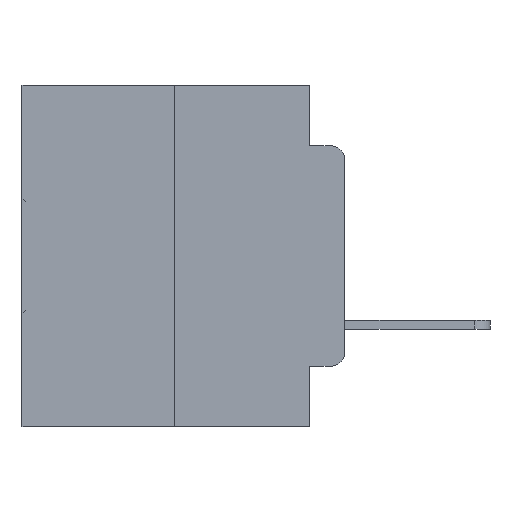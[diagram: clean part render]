
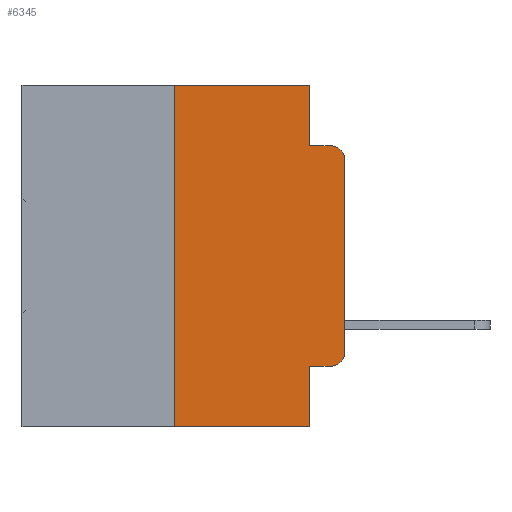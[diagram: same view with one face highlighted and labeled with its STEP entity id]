
A CAD part, left-side view. The second image highlights one B-rep face of the part: STEP entity #6345.
In plain terms, the highlighted planar face has unit normal (-1, 0, 0).
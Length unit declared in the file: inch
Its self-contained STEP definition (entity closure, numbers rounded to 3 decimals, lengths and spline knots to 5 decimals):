
#619 = VECTOR ( 'NONE', #29872, 39.37008 ) ;
#1497 = LINE ( 'NONE', #9899, #13523 ) ;
#1854 = CARTESIAN_POINT ( 'NONE',  ( 0., 0.051, 0. ) ) ;
#1888 = LINE ( 'NONE', #17918, #14671 ) ;
#1907 = LINE ( 'NONE', #19699, #21038 ) ;
#2262 = AXIS2_PLACEMENT_3D ( 'NONE', #8874, #25663, #11394 ) ;
#2297 = VERTEX_POINT ( 'NONE', #15296 ) ;
#3124 = CIRCLE ( 'NONE', #2262, 0.02 ) ;
#3326 = DIRECTION ( 'NONE',  ( 0., 0., -1. ) ) ;
#3469 = ORIENTED_EDGE ( 'NONE', *, *, #19049, .F. ) ;
#3562 = CARTESIAN_POINT ( 'NONE',  ( 0., 0.02, -0.0885 ) ) ;
#5231 = CARTESIAN_POINT ( 'NONE',  ( 0., 0., -0.3915 ) ) ;
#5654 = CARTESIAN_POINT ( 'NONE',  ( 0., 0.051, -0.0885 ) ) ;
#5661 = DIRECTION ( 'NONE',  ( 1., 0., 0. ) ) ;
#6345 = ADVANCED_FACE ( 'NONE', ( #7592 ), #18008, .F. ) ;
#6910 = CARTESIAN_POINT ( 'NONE',  ( 0., 0.25, -0.5 ) ) ;
#7188 = VERTEX_POINT ( 'NONE', #1854 ) ;
#7385 = DIRECTION ( 'NONE',  ( 0., 0., 1. ) ) ;
#7592 = FACE_OUTER_BOUND ( 'NONE', #28493, .T. ) ;
#7648 = LINE ( 'NONE', #8805, #619 ) ;
#7826 = CARTESIAN_POINT ( 'NONE',  ( 0., 0.051, -0.5 ) ) ;
#7956 = LINE ( 'NONE', #9304, #26306 ) ;
#8029 = ORIENTED_EDGE ( 'NONE', *, *, #19196, .F. ) ;
#8427 = ORIENTED_EDGE ( 'NONE', *, *, #16736, .T. ) ;
#8770 = DIRECTION ( 'NONE',  ( 0., -1., 0. ) ) ;
#8805 = CARTESIAN_POINT ( 'NONE',  ( 0., 0.051, -0.0885 ) ) ;
#8874 = CARTESIAN_POINT ( 'NONE',  ( 0., 0.02, -0.3915 ) ) ;
#9270 = DIRECTION ( 'NONE',  ( -1., 0., 0. ) ) ;
#9304 = CARTESIAN_POINT ( 'NONE',  ( 0., 0.473, 0. ) ) ;
#9899 = CARTESIAN_POINT ( 'NONE',  ( 0., 0.051, 0. ) ) ;
#10017 = ORIENTED_EDGE ( 'NONE', *, *, #19286, .F. ) ;
#10334 = VERTEX_POINT ( 'NONE', #21685 ) ;
#11394 = DIRECTION ( 'NONE',  ( 0., 0., -1. ) ) ;
#11712 = VECTOR ( 'NONE', #8770, 39.37008 ) ;
#13026 = DIRECTION ( 'NONE',  ( 0., 0., 1. ) ) ;
#13461 = DIRECTION ( 'NONE',  ( 0., -1., 0. ) ) ;
#13523 = VECTOR ( 'NONE', #24412, 39.37008 ) ;
#13687 = CARTESIAN_POINT ( 'NONE',  ( 0., 0.473, -0.5 ) ) ;
#13739 = VERTEX_POINT ( 'NONE', #20071 ) ;
#14671 = VECTOR ( 'NONE', #13026, 39.37008 ) ;
#14996 = EDGE_CURVE ( 'NONE', #10334, #7188, #7956, .T. ) ;
#15296 = CARTESIAN_POINT ( 'NONE',  ( 0., 0., -0.1085 ) ) ;
#16200 = ORIENTED_EDGE ( 'NONE', *, *, #19373, .T. ) ;
#16364 = ORIENTED_EDGE ( 'NONE', *, *, #18334, .T. ) ;
#16550 = VECTOR ( 'NONE', #13461, 39.37008 ) ;
#16667 = AXIS2_PLACEMENT_3D ( 'NONE', #23773, #9270, #26000 ) ;
#16736 = EDGE_CURVE ( 'NONE', #29200, #27399, #30792, .T. ) ;
#17242 = ORIENTED_EDGE ( 'NONE', *, *, #14996, .F. ) ;
#17918 = CARTESIAN_POINT ( 'NONE',  ( 0., 0.25, 0. ) ) ;
#18008 = PLANE ( 'NONE',  #28939 ) ;
#18196 = EDGE_CURVE ( 'NONE', #27383, #2297, #1907, .T. ) ;
#18315 = CARTESIAN_POINT ( 'NONE',  ( 0., 0.051, 0. ) ) ;
#18334 = EDGE_CURVE ( 'NONE', #2297, #19359, #23637, .T. ) ;
#18565 = ORIENTED_EDGE ( 'NONE', *, *, #18196, .T. ) ;
#18783 = EDGE_CURVE ( 'NONE', #28816, #19359, #7648, .T. ) ;
#19049 = EDGE_CURVE ( 'NONE', #7188, #28816, #1497, .T. ) ;
#19196 = EDGE_CURVE ( 'NONE', #29200, #10334, #1888, .T. ) ;
#19286 = EDGE_CURVE ( 'NONE', #20617, #27399, #30022, .T. ) ;
#19330 = EDGE_CURVE ( 'NONE', #20617, #13739, #28707, .T. ) ;
#19359 = VERTEX_POINT ( 'NONE', #3562 ) ;
#19373 = EDGE_CURVE ( 'NONE', #13739, #27383, #3124, .T. ) ;
#19699 = CARTESIAN_POINT ( 'NONE',  ( 0., 0., 0. ) ) ;
#20071 = CARTESIAN_POINT ( 'NONE',  ( 0., 0.02, -0.4115 ) ) ;
#20258 = CARTESIAN_POINT ( 'NONE',  ( 0., 0.051, -0.4115 ) ) ;
#20617 = VERTEX_POINT ( 'NONE', #20258 ) ;
#21038 = VECTOR ( 'NONE', #7385, 39.37008 ) ;
#21562 = ORIENTED_EDGE ( 'NONE', *, *, #18783, .F. ) ;
#21685 = CARTESIAN_POINT ( 'NONE',  ( 0., 0.25, 0. ) ) ;
#22782 = DIRECTION ( 'NONE',  ( 0., 0., -1. ) ) ;
#23637 = CIRCLE ( 'NONE', #16667, 0.02 ) ;
#23773 = CARTESIAN_POINT ( 'NONE',  ( 0., 0.02, -0.1085 ) ) ;
#24321 = VECTOR ( 'NONE', #3326, 39.37008 ) ;
#24412 = DIRECTION ( 'NONE',  ( 0., 0., -1. ) ) ;
#25663 = DIRECTION ( 'NONE',  ( -1., 0., 0. ) ) ;
#26000 = DIRECTION ( 'NONE',  ( 0., 0., -1. ) ) ;
#26306 = VECTOR ( 'NONE', #30276, 39.37008 ) ;
#27068 = ORIENTED_EDGE ( 'NONE', *, *, #19330, .T. ) ;
#27383 = VERTEX_POINT ( 'NONE', #5231 ) ;
#27399 = VERTEX_POINT ( 'NONE', #7826 ) ;
#28493 = EDGE_LOOP ( 'NONE', ( #18565, #16364, #21562, #3469, #17242, #8029, #8427, #10017, #27068, #16200 ) ) ;
#28707 = LINE ( 'NONE', #29548, #16550 ) ;
#28816 = VERTEX_POINT ( 'NONE', #5654 ) ;
#28939 = AXIS2_PLACEMENT_3D ( 'NONE', #29263, #5661, #22782 ) ;
#29200 = VERTEX_POINT ( 'NONE', #6910 ) ;
#29263 = CARTESIAN_POINT ( 'NONE',  ( 0., 0.473, 0. ) ) ;
#29548 = CARTESIAN_POINT ( 'NONE',  ( 0., 0.051, -0.4115 ) ) ;
#29872 = DIRECTION ( 'NONE',  ( 0., -1., 0. ) ) ;
#30022 = LINE ( 'NONE', #18315, #24321 ) ;
#30276 = DIRECTION ( 'NONE',  ( 0., -1., 0. ) ) ;
#30792 = LINE ( 'NONE', #13687, #11712 ) ;
